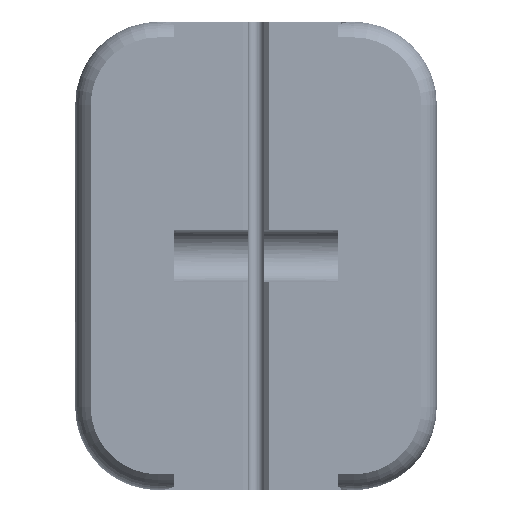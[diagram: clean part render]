
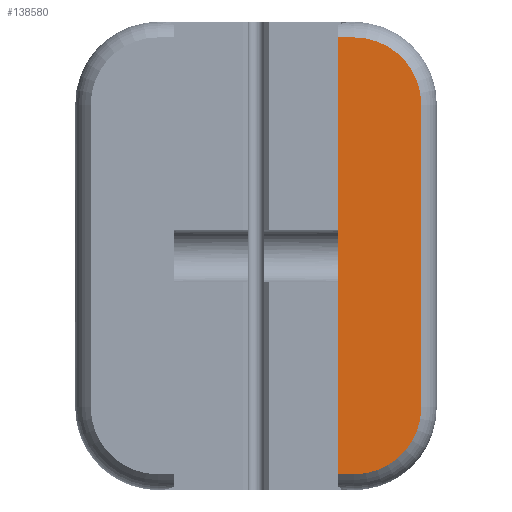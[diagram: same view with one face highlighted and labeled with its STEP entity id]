
A CAD part, top view. The second image highlights one B-rep face of the part: STEP entity #138580.
In plain terms, the highlighted planar face has unit normal (0, 0, 1).
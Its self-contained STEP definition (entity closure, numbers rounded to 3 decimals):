
#20931=PLANE('',#140050);
#28619=FACE_OUTER_BOUND('',#36945,.T.);
#36945=EDGE_LOOP('',(#128875,#128876,#128877,#128878,#128879,#128880));
#37229=CIRCLE('',#140051,6.5);
#37230=CIRCLE('',#140052,6.5);
#45053=LINE('',#313940,#52844);
#45054=LINE('',#313942,#52845);
#45055=LINE('',#313944,#52846);
#45056=LINE('',#313948,#52847);
#52844=VECTOR('',#150542,10.);
#52845=VECTOR('',#150543,10.);
#52846=VECTOR('',#150544,10.);
#52847=VECTOR('',#150547,10.);
#66614=VERTEX_POINT('',#313938);
#66615=VERTEX_POINT('',#313939);
#66616=VERTEX_POINT('',#313941);
#66617=VERTEX_POINT('',#313943);
#66618=VERTEX_POINT('',#313945);
#66619=VERTEX_POINT('',#313947);
#87636=EDGE_CURVE('',#66614,#66615,#45053,.T.);
#87637=EDGE_CURVE('',#66614,#66616,#45054,.T.);
#87638=EDGE_CURVE('',#66617,#66616,#45055,.T.);
#87639=EDGE_CURVE('',#66618,#66617,#37229,.T.);
#87640=EDGE_CURVE('',#66619,#66618,#45056,.T.);
#87641=EDGE_CURVE('',#66615,#66619,#37230,.T.);
#128875=ORIENTED_EDGE('',*,*,#87636,.F.);
#128876=ORIENTED_EDGE('',*,*,#87637,.T.);
#128877=ORIENTED_EDGE('',*,*,#87638,.F.);
#128878=ORIENTED_EDGE('',*,*,#87639,.F.);
#128879=ORIENTED_EDGE('',*,*,#87640,.F.);
#128880=ORIENTED_EDGE('',*,*,#87641,.F.);
#138580=ADVANCED_FACE('',(#28619),#20931,.F.);
#140050=AXIS2_PLACEMENT_3D('',#313937,#150540,#150541);
#140051=AXIS2_PLACEMENT_3D('',#313946,#150545,#150546);
#140052=AXIS2_PLACEMENT_3D('',#313949,#150548,#150549);
#150540=DIRECTION('center_axis',(0.,0.,
-1.));
#150541=DIRECTION('ref_axis',(1.,0.,0.));
#150542=DIRECTION('',(1.,0.,0.));
#150543=DIRECTION('',(0.,-1.,0.));
#150544=DIRECTION('',(-1.,0.,0.));
#150545=DIRECTION('center_axis',(0.,0.,
-1.));
#150546=DIRECTION('ref_axis',(0.707,-0.707,0.));
#150547=DIRECTION('',(0.,-1.,0.));
#150548=DIRECTION('center_axis',(0.,0.,
-1.));
#150549=DIRECTION('ref_axis',(0.707,0.707,0.));
#313937=CARTESIAN_POINT('Origin',(-20.269,69.903,-24.354));
#313938=CARTESIAN_POINT('',(7.936,76.153,-24.354));
#313939=CARTESIAN_POINT('',(9.5,76.153,-24.354));
#313940=CARTESIAN_POINT('',(-10.135,76.153,-24.354));
#313941=CARTESIAN_POINT('',(7.936,33.855,-24.354));
#313942=CARTESIAN_POINT('',(7.936,42.504,-24.354));
#313943=CARTESIAN_POINT('',(9.5,33.855,-24.354));
#313944=CARTESIAN_POINT('',(-10.135,33.855,-24.354));
#313945=CARTESIAN_POINT('',(16.,40.355,-24.354));
#313946=CARTESIAN_POINT('Origin',(9.5,40.355,-24.354));
#313947=CARTESIAN_POINT('',(16.,69.653,-24.354));
#313948=CARTESIAN_POINT('',(16.,69.903,-24.354));
#313949=CARTESIAN_POINT('Origin',(9.5,69.653,-24.354));
